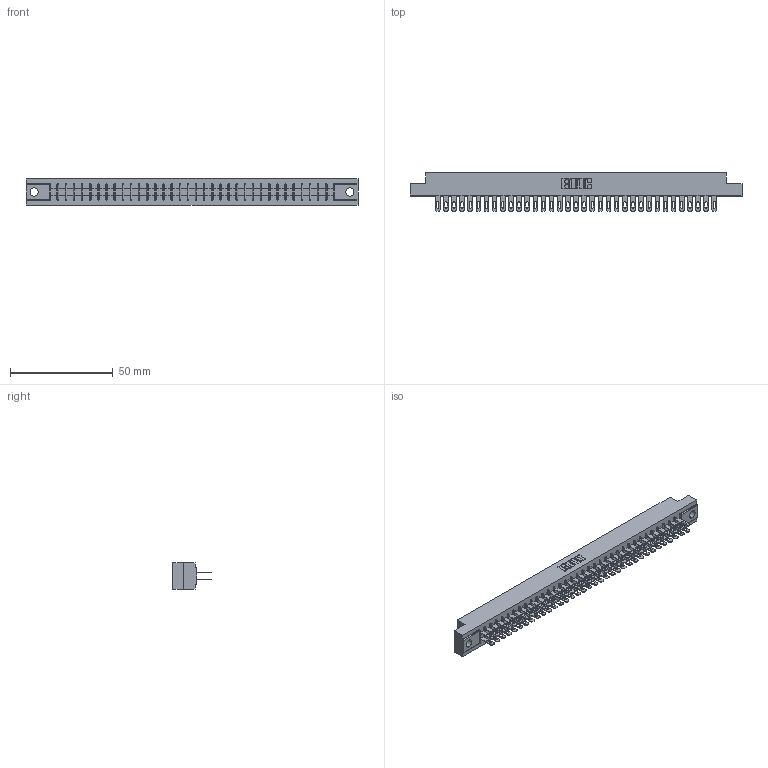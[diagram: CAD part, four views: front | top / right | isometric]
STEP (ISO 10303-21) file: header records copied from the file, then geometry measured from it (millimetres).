
FILE_DESCRIPTION (( 'STEP AP203' ), '1' );
FILE_NAME ('305-070-500-504.STEP', '2019-09-10T04:59:31', ( '' ), ( '' ), 'SwSTEP 2.0', 'SolidWorks 2016', '' );
FILE_SCHEMA (( 'CONFIG_CONTROL_DESIGN' ));
Length unit declared in the file: inch
Products named in the file (3): 305-290-001_500; 305-070-500-504; 305 Part_.156 Dia
Assembly tree (71 placements, depth 2):
  305-070-500-504
    305 Part_.156 Dia
    305-290-001_500  x70
Bounding box: 161.7 x 18.85 x 12.7 mm (x, y, z)
Volume: 16452.7 mm3; surface area: 22756.7 mm2
Topology: 71 solids, 71 shells, 3630 faces, 10397 edges, 6742 vertices
Faces by surface type: plane 2042, cylinder 1448, sphere 140
Entity records: 39188 total; most frequent: CARTESIAN_POINT 6489, ORIENTED_EDGE 6438, DIRECTION 6277, EDGE_CURVE 3219, LINE 2601, VECTOR 2601, VERTEX_POINT 2050, AXIS2_PLACEMENT_3D 1838
